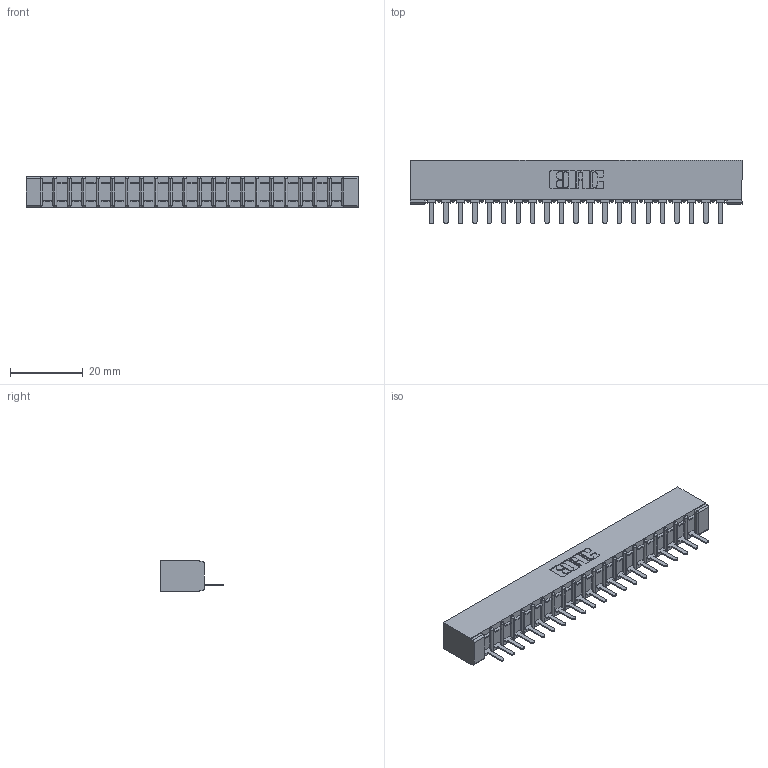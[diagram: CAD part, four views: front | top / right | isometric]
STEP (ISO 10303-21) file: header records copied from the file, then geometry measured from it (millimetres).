
FILE_DESCRIPTION (( 'STEP AP203' ), '1' );
FILE_NAME ('357-021-521-101.STEP', '2019-09-16T22:40:17', ( '' ), ( '' ), 'SwSTEP 2.0', 'SolidWorks 2016', '' );
FILE_SCHEMA (( 'CONFIG_CONTROL_DESIGN' ));
Length unit declared in the file: inch
Products named in the file (3): 307-290-002_521; 307 Part_No Mounting Lugs; 357-021-521-101
Assembly tree (22 placements, depth 2):
  357-021-521-101
    307 Part_No Mounting Lugs
    307-290-002_521  x21
Bounding box: 91.08 x 17.42 x 8.71 mm (x, y, z)
Volume: 6256.2 mm3; surface area: 11843.2 mm2
Topology: 22 solids, 22 shells, 1686 faces, 5171 edges, 3386 vertices
Faces by surface type: plane 1011, cylinder 631, sphere 44
Entity records: 21032 total; most frequent: CARTESIAN_POINT 3544, ORIENTED_EDGE 3534, DIRECTION 3451, EDGE_CURVE 1767, VECTOR 1345, LINE 1345, VERTEX_POINT 1146, AXIS2_PLACEMENT_3D 1053
